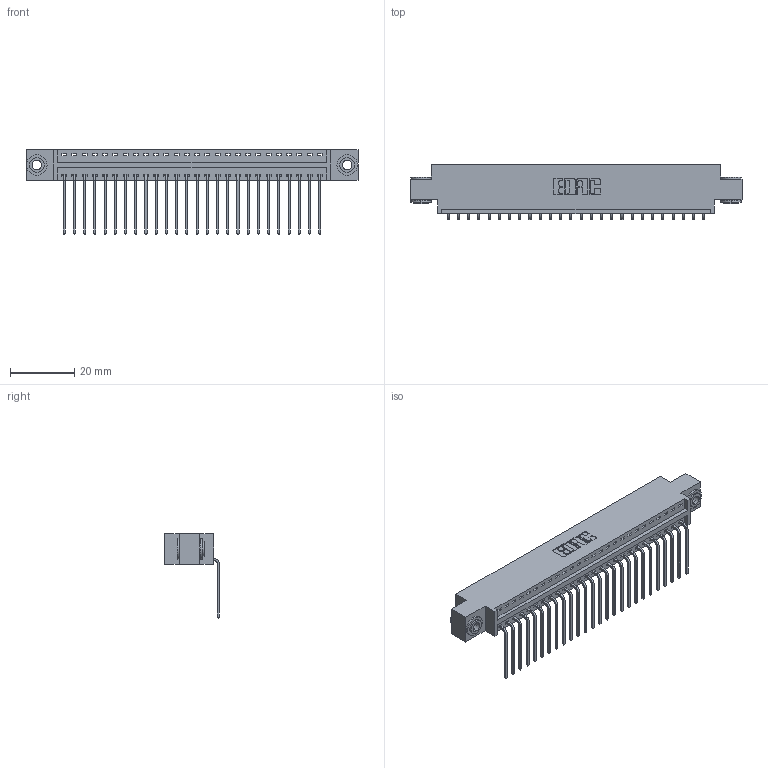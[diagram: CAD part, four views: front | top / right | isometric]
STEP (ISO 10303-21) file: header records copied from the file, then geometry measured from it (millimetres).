
FILE_DESCRIPTION (( 'STEP AP203' ), '1' );
FILE_NAME ('346-026-559-603.STEP', '2022-05-06T03:39:28', ( '' ), ( '' ), 'SwSTEP 2.0', 'SolidWorks 2020', '' );
FILE_SCHEMA (( 'CONFIG_CONTROL_DESIGN' ));
Length unit declared in the file: inch
Products named in the file (4): 346-026-559-603; 345-292-001_558 559 Tail - 1; 345-250-002_345-250-002-102; 346 Part_0.170 Offset - 0.156 Dia-TH
Assembly tree (29 placements, depth 2):
  346-026-559-603
    346 Part_0.170 Offset - 0.156 Dia-TH
    345-292-001_558 559 Tail - 1  x26
    345-250-002_345-250-002-102  x2
Bounding box: 103.12 x 17.08 x 26.16 mm (x, y, z)
Volume: 9694.3 mm3; surface area: 12872.6 mm2
Topology: 29 solids, 29 shells, 1738 faces, 5185 edges, 3418 vertices
Faces by surface type: plane 1196, cylinder 534, cone 8
Entity records: 19572 total; most frequent: CARTESIAN_POINT 3343, ORIENTED_EDGE 3294, DIRECTION 2997, EDGE_CURVE 1647, LINE 1387, VECTOR 1387, VERTEX_POINT 1094, AXIS2_PLACEMENT_3D 805
